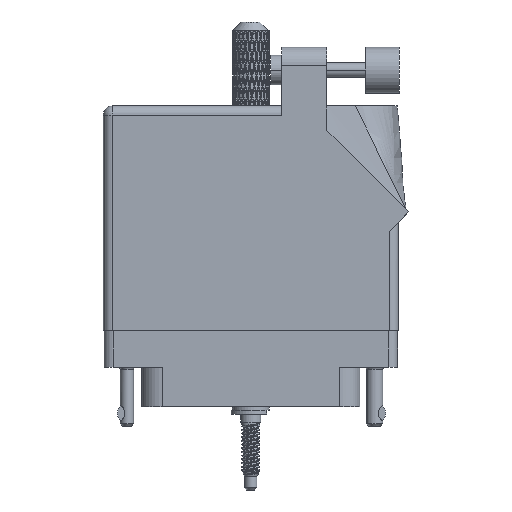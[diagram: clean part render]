
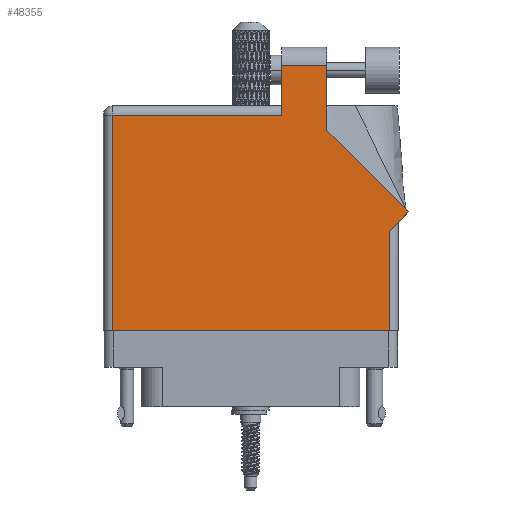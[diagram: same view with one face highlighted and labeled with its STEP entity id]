
A CAD part, front view. The second image highlights one B-rep face of the part: STEP entity #48355.
In plain terms, the highlighted face is planar.
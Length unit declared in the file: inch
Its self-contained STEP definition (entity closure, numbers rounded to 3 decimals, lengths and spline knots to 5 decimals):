
#2844 = EDGE_CURVE ( 'NONE', #28794, #112326, #86010, .T. ) ;
#4204 = EDGE_LOOP ( 'NONE', ( #76235, #87372, #12090, #112482, #70560, #15522, #113378, #100261, #97670 ) ) ;
#6773 = DIRECTION ( 'NONE',  ( -1., 0., 0. ) ) ;
#8771 = CARTESIAN_POINT ( 'NONE',  ( 0.212, 1.705, 0.455 ) ) ;
#9779 = DIRECTION ( 'NONE',  ( -1., 0., 0. ) ) ;
#12090 = ORIENTED_EDGE ( 'NONE', *, *, #33588, .T. ) ;
#15229 = CARTESIAN_POINT ( 'NONE',  ( 0.519, 1.26442, 0.455 ) ) ;
#15522 = ORIENTED_EDGE ( 'NONE', *, *, #113955, .T. ) ;
#17451 = EDGE_CURVE ( 'NONE', #112326, #79025, #59337, .T. ) ;
#18934 = VERTEX_POINT ( 'NONE', #34484 ) ;
#20115 = LINE ( 'NONE', #15229, #36608 ) ;
#21775 = VERTEX_POINT ( 'NONE', #79753 ) ;
#23448 = CARTESIAN_POINT ( 'NONE',  ( -1.005, 1.368, 0.455 ) ) ;
#26542 = LINE ( 'NONE', #84755, #76579 ) ;
#26667 = VECTOR ( 'NONE', #98473, 39.37008 ) ;
#27589 = DIRECTION ( 'NONE',  ( -1., 0., 0. ) ) ;
#28584 = VECTOR ( 'NONE', #33865, 39.37008 ) ;
#28794 = VERTEX_POINT ( 'NONE', #54165 ) ;
#29779 = EDGE_CURVE ( 'NONE', #67979, #28794, #68550, .T. ) ;
#31304 = EDGE_CURVE ( 'NONE', #107217, #21775, #40646, .T. ) ;
#31465 = FACE_OUTER_BOUND ( 'NONE', #4204, .T. ) ;
#32095 = CARTESIAN_POINT ( 'NONE',  ( 1.07571, 0.70771, 0.455 ) ) ;
#33474 = CARTESIAN_POINT ( 'NONE',  ( -1.005, -0.1, 0.455 ) ) ;
#33588 = EDGE_CURVE ( 'NONE', #42812, #18934, #26542, .T. ) ;
#33865 = DIRECTION ( 'NONE',  ( 1., 0., 0. ) ) ;
#34441 = CARTESIAN_POINT ( 'NONE',  ( 0.519, 1.26442, 0.455 ) ) ;
#34484 = CARTESIAN_POINT ( 'NONE',  ( 0.212, 1.368, 0.455 ) ) ;
#34774 = EDGE_CURVE ( 'NONE', #89222, #42812, #59720, .T. ) ;
#35696 = VECTOR ( 'NONE', #40708, 39.37008 ) ;
#36608 = VECTOR ( 'NONE', #86188, 39.37008 ) ;
#40646 = LINE ( 'NONE', #107722, #26667 ) ;
#40708 = DIRECTION ( 'NONE',  ( -0.707, 0.707, 0. ) ) ;
#42812 = VERTEX_POINT ( 'NONE', #8771 ) ;
#44761 = CARTESIAN_POINT ( 'NONE',  ( -1.005, 1.43, 0.455 ) ) ;
#48061 = DIRECTION ( 'NONE',  ( 0., 1., 0. ) ) ;
#48355 = ADVANCED_FACE ( 'NONE', ( #31465 ), #61804, .F. ) ;
#51295 = VECTOR ( 'NONE', #76833, 39.37008 ) ;
#54165 = CARTESIAN_POINT ( 'NONE',  ( 0.943, 0.575, 0.455 ) ) ;
#59337 = LINE ( 'NONE', #32095, #35696 ) ;
#59720 = LINE ( 'NONE', #71005, #75034 ) ;
#61500 = CARTESIAN_POINT ( 'NONE',  ( 0.943, -0.1, 0.455 ) ) ;
#61804 = PLANE ( 'NONE',  #83415 ) ;
#62490 = EDGE_CURVE ( 'NONE', #18934, #107217, #79911, .T. ) ;
#67979 = VERTEX_POINT ( 'NONE', #61500 ) ;
#68550 = LINE ( 'NONE', #110863, #89351 ) ;
#70560 = ORIENTED_EDGE ( 'NONE', *, *, #31304, .T. ) ;
#71005 = CARTESIAN_POINT ( 'NONE',  ( 0.212, 1.705, 0.455 ) ) ;
#75034 = VECTOR ( 'NONE', #9779, 39.37008 ) ;
#76041 = EDGE_CURVE ( 'NONE', #79025, #89222, #20115, .T. ) ;
#76235 = ORIENTED_EDGE ( 'NONE', *, *, #76041, .T. ) ;
#76579 = VECTOR ( 'NONE', #78879, 39.37008 ) ;
#76833 = DIRECTION ( 'NONE',  ( 0.707, 0.707, 0. ) ) ;
#78879 = DIRECTION ( 'NONE',  ( 0., -1., 0. ) ) ;
#79025 = VERTEX_POINT ( 'NONE', #34441 ) ;
#79753 = CARTESIAN_POINT ( 'NONE',  ( -0.943, -0.1, 0.455 ) ) ;
#79911 = LINE ( 'NONE', #23448, #107582 ) ;
#83415 = AXIS2_PLACEMENT_3D ( 'NONE', #44761, #106768, #27589 ) ;
#83509 = CARTESIAN_POINT ( 'NONE',  ( -0.943, 1.368, 0.455 ) ) ;
#83836 = CARTESIAN_POINT ( 'NONE',  ( 1.07571, 0.70771, 0.455 ) ) ;
#84755 = CARTESIAN_POINT ( 'NONE',  ( 0.212, 1.43, 0.455 ) ) ;
#86010 = LINE ( 'NONE', #103903, #51295 ) ;
#86188 = DIRECTION ( 'NONE',  ( 0., 1., 0. ) ) ;
#87372 = ORIENTED_EDGE ( 'NONE', *, *, #34774, .T. ) ;
#89222 = VERTEX_POINT ( 'NONE', #111769 ) ;
#89351 = VECTOR ( 'NONE', #48061, 39.37008 ) ;
#96662 = LINE ( 'NONE', #33474, #28584 ) ;
#97670 = ORIENTED_EDGE ( 'NONE', *, *, #17451, .T. ) ;
#98473 = DIRECTION ( 'NONE',  ( 0., -1., 0. ) ) ;
#100261 = ORIENTED_EDGE ( 'NONE', *, *, #2844, .T. ) ;
#103903 = CARTESIAN_POINT ( 'NONE',  ( 1.005, 0.637, 0.455 ) ) ;
#106768 = DIRECTION ( 'NONE',  ( 0., 0., -1. ) ) ;
#107217 = VERTEX_POINT ( 'NONE', #83509 ) ;
#107582 = VECTOR ( 'NONE', #6773, 39.37008 ) ;
#107722 = CARTESIAN_POINT ( 'NONE',  ( -0.943, -0.1, 0.455 ) ) ;
#110863 = CARTESIAN_POINT ( 'NONE',  ( 0.943, 0.637, 0.455 ) ) ;
#111769 = CARTESIAN_POINT ( 'NONE',  ( 0.519, 1.705, 0.455 ) ) ;
#112326 = VERTEX_POINT ( 'NONE', #83836 ) ;
#112482 = ORIENTED_EDGE ( 'NONE', *, *, #62490, .T. ) ;
#113378 = ORIENTED_EDGE ( 'NONE', *, *, #29779, .T. ) ;
#113955 = EDGE_CURVE ( 'NONE', #21775, #67979, #96662, .T. ) ;
